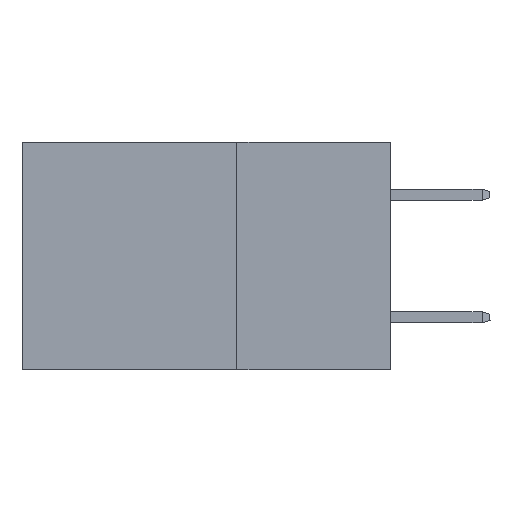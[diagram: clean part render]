
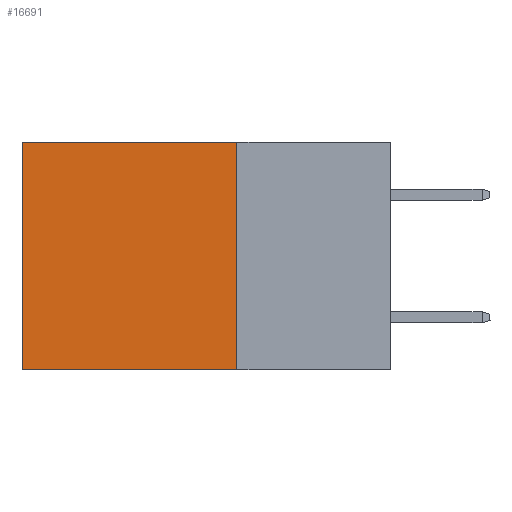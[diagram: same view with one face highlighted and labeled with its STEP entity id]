
A CAD part, left-side view. The second image highlights one B-rep face of the part: STEP entity #16691.
In plain terms, the highlighted planar face has unit normal (-1, 0, 0).
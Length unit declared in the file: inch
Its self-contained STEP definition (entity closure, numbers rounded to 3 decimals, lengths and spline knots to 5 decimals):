
#975 = DIRECTION ( 'NONE',  ( 0., 0., -1. ) ) ;
#1073 = AXIS2_PLACEMENT_3D ( 'NONE', #25996, #7617, #25053 ) ;
#4378 = ORIENTED_EDGE ( 'NONE', *, *, #6297, .T. ) ;
#6297 = EDGE_CURVE ( 'NONE', #43781, #26922, #36776, .T. ) ;
#6506 = CARTESIAN_POINT ( 'NONE',  ( 0.2875, 0.6, 0. ) ) ;
#7617 = DIRECTION ( 'NONE',  ( 1., 0., 0. ) ) ;
#8616 = CARTESIAN_POINT ( 'NONE',  ( 0.2875, 0.25, -0.37 ) ) ;
#9591 = LINE ( 'NONE', #44664, #14910 ) ;
#11398 = VECTOR ( 'NONE', #975, 39.37008 ) ;
#12846 = LINE ( 'NONE', #34023, #45091 ) ;
#14288 = VECTOR ( 'NONE', #33115, 39.37008 ) ;
#14910 = VECTOR ( 'NONE', #20429, 39.37008 ) ;
#15287 = CARTESIAN_POINT ( 'NONE',  ( 0.2875, 0.25, -0.37 ) ) ;
#16138 = DIRECTION ( 'NONE',  ( 0., 1., 0. ) ) ;
#16691 = ADVANCED_FACE ( 'NONE', ( #28596 ), #35877, .F. ) ;
#20429 = DIRECTION ( 'NONE',  ( 0., 0., -1. ) ) ;
#21258 = EDGE_CURVE ( 'NONE', #44890, #40240, #9591, .T. ) ;
#24871 = EDGE_CURVE ( 'NONE', #44890, #43781, #12846, .T. ) ;
#25053 = DIRECTION ( 'NONE',  ( 0., 0., -1. ) ) ;
#25996 = CARTESIAN_POINT ( 'NONE',  ( 0.2875, 0.25, 0. ) ) ;
#26639 = CARTESIAN_POINT ( 'NONE',  ( 0.2875, 0.6, -0.37 ) ) ;
#26922 = VERTEX_POINT ( 'NONE', #26639 ) ;
#28023 = ORIENTED_EDGE ( 'NONE', *, *, #39219, .F. ) ;
#28596 = FACE_OUTER_BOUND ( 'NONE', #45142, .T. ) ;
#30554 = CARTESIAN_POINT ( 'NONE',  ( 0.2875, 0.25, 0. ) ) ;
#33115 = DIRECTION ( 'NONE',  ( 0., 1., 0. ) ) ;
#33237 = CARTESIAN_POINT ( 'NONE',  ( 0.2875, 0.6, 0. ) ) ;
#34023 = CARTESIAN_POINT ( 'NONE',  ( 0.2875, 0.25, 0. ) ) ;
#35877 = PLANE ( 'NONE',  #1073 ) ;
#36776 = LINE ( 'NONE', #33237, #11398 ) ;
#39219 = EDGE_CURVE ( 'NONE', #40240, #26922, #40400, .T. ) ;
#39314 = ORIENTED_EDGE ( 'NONE', *, *, #21258, .F. ) ;
#40240 = VERTEX_POINT ( 'NONE', #15287 ) ;
#40400 = LINE ( 'NONE', #8616, #14288 ) ;
#43781 = VERTEX_POINT ( 'NONE', #6506 ) ;
#43992 = ORIENTED_EDGE ( 'NONE', *, *, #24871, .T. ) ;
#44664 = CARTESIAN_POINT ( 'NONE',  ( 0.2875, 0.25, 0. ) ) ;
#44890 = VERTEX_POINT ( 'NONE', #30554 ) ;
#45091 = VECTOR ( 'NONE', #16138, 39.37008 ) ;
#45142 = EDGE_LOOP ( 'NONE', ( #4378, #28023, #39314, #43992 ) ) ;
